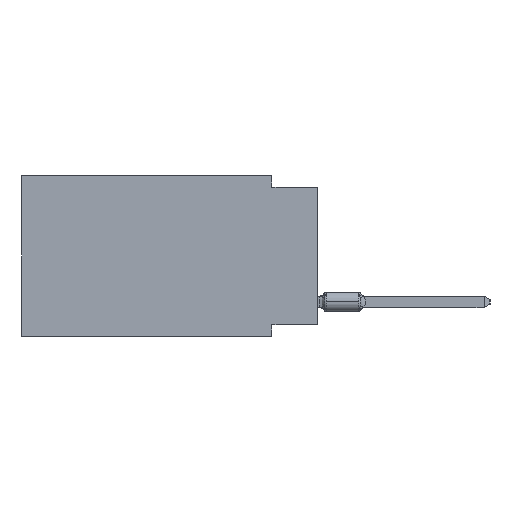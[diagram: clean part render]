
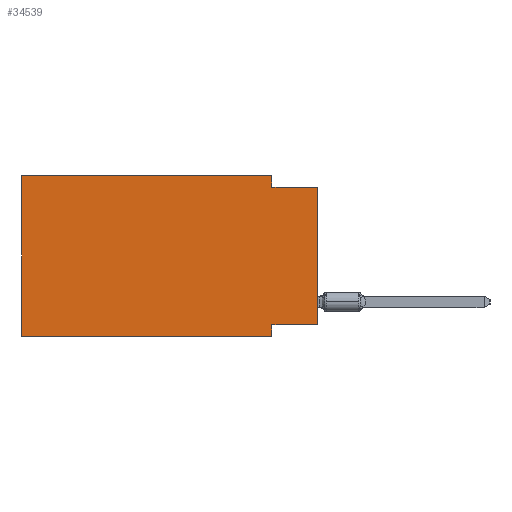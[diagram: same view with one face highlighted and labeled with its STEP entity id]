
A CAD part, left-side view. The second image highlights one B-rep face of the part: STEP entity #34539.
In plain terms, the highlighted planar face has unit normal (-1, 0, 0).
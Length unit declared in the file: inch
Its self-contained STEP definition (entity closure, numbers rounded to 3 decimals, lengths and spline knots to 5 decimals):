
#41 = DIRECTION ( 'NONE',  ( 0., 0., -1. ) ) ;
#86 = VERTEX_POINT ( 'NONE', #38103 ) ;
#883 = CARTESIAN_POINT ( 'NONE',  ( 0., 0.1, 0. ) ) ;
#1117 = EDGE_CURVE ( 'NONE', #25570, #21995, #32849, .T. ) ;
#1501 = LINE ( 'NONE', #37659, #38501 ) ;
#1775 = VERTEX_POINT ( 'NONE', #16369 ) ;
#1806 = LINE ( 'NONE', #7151, #26010 ) ;
#2379 = ORIENTED_EDGE ( 'NONE', *, *, #28371, .F. ) ;
#3345 = FACE_OUTER_BOUND ( 'NONE', #31755, .T. ) ;
#4537 = EDGE_CURVE ( 'NONE', #32023, #36684, #21843, .T. ) ;
#6193 = VECTOR ( 'NONE', #33615, 39.37008 ) ;
#7151 = CARTESIAN_POINT ( 'NONE',  ( 0., 0., 0. ) ) ;
#7318 = CARTESIAN_POINT ( 'NONE',  ( 0., 0.1, -0.025 ) ) ;
#7461 = DIRECTION ( 'NONE',  ( 0., 0., 1. ) ) ;
#8071 = CARTESIAN_POINT ( 'NONE',  ( 0., 0., -0.325 ) ) ;
#8582 = CARTESIAN_POINT ( 'NONE',  ( 0., 0., -0.025 ) ) ;
#8780 = CARTESIAN_POINT ( 'NONE',  ( 0., 0.645, 0. ) ) ;
#8883 = PLANE ( 'NONE',  #24861 ) ;
#10592 = DIRECTION ( 'NONE',  ( 0., -1., 0. ) ) ;
#12082 = LINE ( 'NONE', #27865, #6193 ) ;
#12316 = CARTESIAN_POINT ( 'NONE',  ( 0., 0.1, 0. ) ) ;
#13256 = VECTOR ( 'NONE', #36051, 39.37008 ) ;
#15402 = DIRECTION ( 'NONE',  ( 0., 0., -1. ) ) ;
#16369 = CARTESIAN_POINT ( 'NONE',  ( 0., 0.1, -0.35 ) ) ;
#16430 = DIRECTION ( 'NONE',  ( 0., 0., 1. ) ) ;
#16506 = EDGE_CURVE ( 'NONE', #31141, #25570, #23792, .T. ) ;
#18273 = LINE ( 'NONE', #27979, #25913 ) ;
#19181 = EDGE_CURVE ( 'NONE', #32023, #21201, #1806, .T. ) ;
#19373 = ORIENTED_EDGE ( 'NONE', *, *, #21737, .F. ) ;
#20737 = CARTESIAN_POINT ( 'NONE',  ( 0., 0.645, 0. ) ) ;
#21201 = VERTEX_POINT ( 'NONE', #8582 ) ;
#21737 = EDGE_CURVE ( 'NONE', #36684, #1775, #12082, .T. ) ;
#21843 = LINE ( 'NONE', #36866, #38811 ) ;
#21995 = VERTEX_POINT ( 'NONE', #7318 ) ;
#22311 = VECTOR ( 'NONE', #41, 39.37008 ) ;
#22438 = DIRECTION ( 'NONE',  ( 0., 1., 0. ) ) ;
#23792 = LINE ( 'NONE', #8780, #13256 ) ;
#24861 = AXIS2_PLACEMENT_3D ( 'NONE', #20737, #38925, #15402 ) ;
#25570 = VERTEX_POINT ( 'NONE', #883 ) ;
#25715 = ORIENTED_EDGE ( 'NONE', *, *, #1117, .F. ) ;
#25913 = VECTOR ( 'NONE', #30360, 39.37008 ) ;
#26010 = VECTOR ( 'NONE', #16430, 39.37008 ) ;
#26107 = CARTESIAN_POINT ( 'NONE',  ( 0., 0.1, -0.325 ) ) ;
#26229 = LINE ( 'NONE', #37880, #35978 ) ;
#26888 = ORIENTED_EDGE ( 'NONE', *, *, #29963, .T. ) ;
#27865 = CARTESIAN_POINT ( 'NONE',  ( 0., 0.1, -0.35 ) ) ;
#27979 = CARTESIAN_POINT ( 'NONE',  ( 0., 0., -0.025 ) ) ;
#28371 = EDGE_CURVE ( 'NONE', #86, #31141, #26229, .T. ) ;
#28747 = EDGE_CURVE ( 'NONE', #21995, #21201, #18273, .T. ) ;
#29963 = EDGE_CURVE ( 'NONE', #86, #1775, #1501, .T. ) ;
#30289 = ORIENTED_EDGE ( 'NONE', *, *, #19181, .T. ) ;
#30360 = DIRECTION ( 'NONE',  ( 0., -1., 0. ) ) ;
#30495 = ORIENTED_EDGE ( 'NONE', *, *, #28747, .F. ) ;
#31141 = VERTEX_POINT ( 'NONE', #37416 ) ;
#31323 = ORIENTED_EDGE ( 'NONE', *, *, #16506, .F. ) ;
#31755 = EDGE_LOOP ( 'NONE', ( #30289, #30495, #25715, #31323, #2379, #26888, #19373, #37234 ) ) ;
#32023 = VERTEX_POINT ( 'NONE', #8071 ) ;
#32849 = LINE ( 'NONE', #12316, #22311 ) ;
#33615 = DIRECTION ( 'NONE',  ( 0., 0., -1. ) ) ;
#34539 = ADVANCED_FACE ( 'NONE', ( #3345 ), #8883, .F. ) ;
#35978 = VECTOR ( 'NONE', #7461, 39.37008 ) ;
#36051 = DIRECTION ( 'NONE',  ( 0., -1., 0. ) ) ;
#36684 = VERTEX_POINT ( 'NONE', #26107 ) ;
#36866 = CARTESIAN_POINT ( 'NONE',  ( 0., 0., -0.325 ) ) ;
#37234 = ORIENTED_EDGE ( 'NONE', *, *, #4537, .F. ) ;
#37416 = CARTESIAN_POINT ( 'NONE',  ( 0., 0.645, 0. ) ) ;
#37659 = CARTESIAN_POINT ( 'NONE',  ( 0., 0.645, -0.35 ) ) ;
#37880 = CARTESIAN_POINT ( 'NONE',  ( 0., 0.645, 0. ) ) ;
#38103 = CARTESIAN_POINT ( 'NONE',  ( 0., 0.645, -0.35 ) ) ;
#38501 = VECTOR ( 'NONE', #10592, 39.37008 ) ;
#38811 = VECTOR ( 'NONE', #22438, 39.37008 ) ;
#38925 = DIRECTION ( 'NONE',  ( 1., 0., 0. ) ) ;
